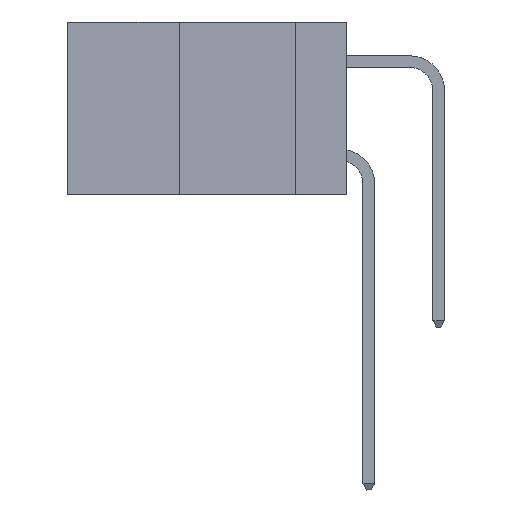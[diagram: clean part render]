
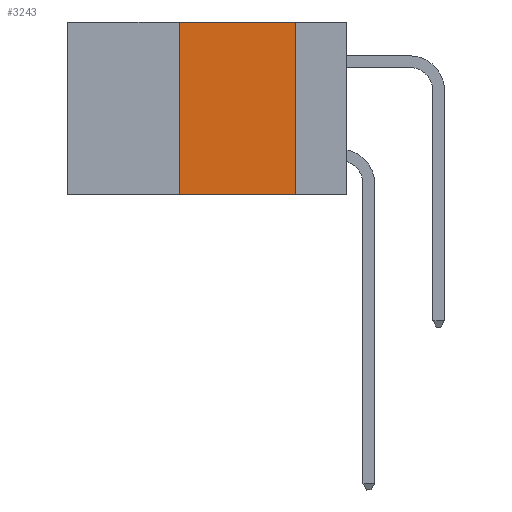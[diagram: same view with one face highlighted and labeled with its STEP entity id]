
A CAD part, left-side view. The second image highlights one B-rep face of the part: STEP entity #3243.
In plain terms, the highlighted planar face has unit normal (-1, 0, 0).
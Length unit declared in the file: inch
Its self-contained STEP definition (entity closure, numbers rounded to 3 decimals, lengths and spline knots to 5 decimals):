
#166 = DIRECTION ( 'NONE',  ( 0., 0., -1. ) ) ;
#356 = AXIS2_PLACEMENT_3D ( 'NONE', #684, #989, #5403 ) ;
#501 = ORIENTED_EDGE ( 'NONE', *, *, #27656, .F. ) ;
#684 = CARTESIAN_POINT ( 'NONE',  ( 0., 0.6, 0. ) ) ;
#989 = DIRECTION ( 'NONE',  ( 1., 0., 0. ) ) ;
#2174 = EDGE_LOOP ( 'NONE', ( #501, #18996, #14536, #11516 ) ) ;
#2898 = CARTESIAN_POINT ( 'NONE',  ( 0., 0.11, 0. ) ) ;
#2974 = CARTESIAN_POINT ( 'NONE',  ( 0., 0.36, 0. ) ) ;
#3243 = ADVANCED_FACE ( 'NONE', ( #16290 ), #14168, .F. ) ;
#5166 = DIRECTION ( 'NONE',  ( 0., -1., 0. ) ) ;
#5403 = DIRECTION ( 'NONE',  ( 0., 0., -1. ) ) ;
#6469 = CARTESIAN_POINT ( 'NONE',  ( 0., 0.11, -0.37 ) ) ;
#6592 = CARTESIAN_POINT ( 'NONE',  ( 0., 0.36, -0.37 ) ) ;
#7414 = CARTESIAN_POINT ( 'NONE',  ( 0., 0.6, -0.37 ) ) ;
#9736 = EDGE_CURVE ( 'NONE', #24724, #11382, #18865, .T. ) ;
#9811 = DIRECTION ( 'NONE',  ( 0., -1., 0. ) ) ;
#9951 = CARTESIAN_POINT ( 'NONE',  ( 0., 0.6, 0. ) ) ;
#11382 = VERTEX_POINT ( 'NONE', #21141 ) ;
#11516 = ORIENTED_EDGE ( 'NONE', *, *, #24351, .T. ) ;
#12335 = LINE ( 'NONE', #9951, #28202 ) ;
#13191 = EDGE_CURVE ( 'NONE', #11382, #21577, #12335, .T. ) ;
#14168 = PLANE ( 'NONE',  #356 ) ;
#14536 = ORIENTED_EDGE ( 'NONE', *, *, #9736, .F. ) ;
#14970 = LINE ( 'NONE', #7414, #18116 ) ;
#16114 = CARTESIAN_POINT ( 'NONE',  ( 0., 0.11, 0. ) ) ;
#16290 = FACE_OUTER_BOUND ( 'NONE', #2174, .T. ) ;
#18116 = VECTOR ( 'NONE', #9811, 39.37008 ) ;
#18332 = VECTOR ( 'NONE', #166, 39.37008 ) ;
#18865 = LINE ( 'NONE', #2974, #23825 ) ;
#18996 = ORIENTED_EDGE ( 'NONE', *, *, #13191, .F. ) ;
#19182 = DIRECTION ( 'NONE',  ( 0., 0., 1. ) ) ;
#21141 = CARTESIAN_POINT ( 'NONE',  ( 0., 0.36, 0. ) ) ;
#21577 = VERTEX_POINT ( 'NONE', #2898 ) ;
#22006 = VERTEX_POINT ( 'NONE', #6469 ) ;
#23825 = VECTOR ( 'NONE', #19182, 39.37008 ) ;
#24351 = EDGE_CURVE ( 'NONE', #24724, #22006, #14970, .T. ) ;
#24724 = VERTEX_POINT ( 'NONE', #6592 ) ;
#25096 = LINE ( 'NONE', #16114, #18332 ) ;
#27656 = EDGE_CURVE ( 'NONE', #21577, #22006, #25096, .T. ) ;
#28202 = VECTOR ( 'NONE', #5166, 39.37008 ) ;
